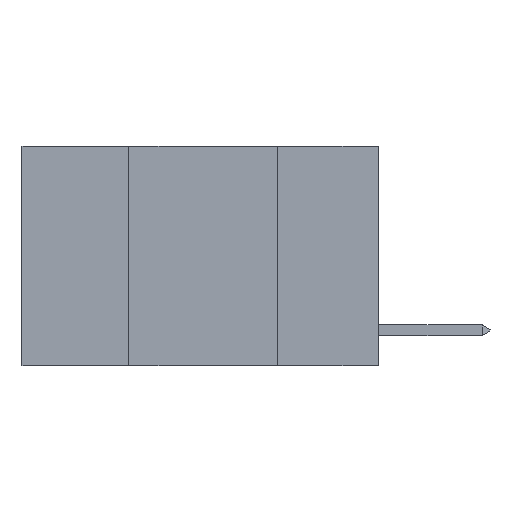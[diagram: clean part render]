
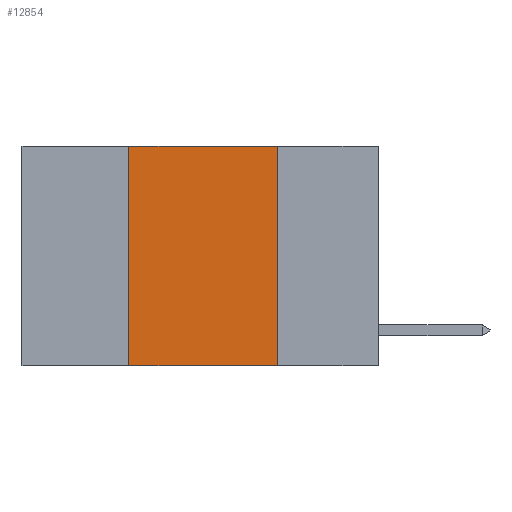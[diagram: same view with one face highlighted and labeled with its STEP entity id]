
A CAD part, left-side view. The second image highlights one B-rep face of the part: STEP entity #12854.
In plain terms, the highlighted planar face has unit normal (-1, 0, 0).
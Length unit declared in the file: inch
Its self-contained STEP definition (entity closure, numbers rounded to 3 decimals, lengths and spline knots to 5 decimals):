
#2386 = LINE ( 'NONE', #8048, #11723 ) ;
#2645 = VECTOR ( 'NONE', #6555, 39.37008 ) ;
#3430 = VERTEX_POINT ( 'NONE', #19271 ) ;
#3603 = VERTEX_POINT ( 'NONE', #8243 ) ;
#4232 = PLANE ( 'NONE',  #12462 ) ;
#4499 = ORIENTED_EDGE ( 'NONE', *, *, #13078, .F. ) ;
#5145 = VERTEX_POINT ( 'NONE', #18875 ) ;
#6231 = CARTESIAN_POINT ( 'NONE',  ( 0., 0.42, 0. ) ) ;
#6555 = DIRECTION ( 'NONE',  ( 0., -1., 0. ) ) ;
#6727 = VECTOR ( 'NONE', #12783, 39.37008 ) ;
#7423 = VECTOR ( 'NONE', #11514, 39.37008 ) ;
#7476 = EDGE_CURVE ( 'NONE', #3430, #5145, #15896, .T. ) ;
#7584 = CARTESIAN_POINT ( 'NONE',  ( 0., 0.6, 0. ) ) ;
#8048 = CARTESIAN_POINT ( 'NONE',  ( 0., 0.6, 0. ) ) ;
#8227 = CARTESIAN_POINT ( 'NONE',  ( 0., 0.6, -0.37 ) ) ;
#8243 = CARTESIAN_POINT ( 'NONE',  ( 0., 0.42, 0. ) ) ;
#8637 = EDGE_CURVE ( 'NONE', #3430, #3603, #18887, .T. ) ;
#9293 = DIRECTION ( 'NONE',  ( 0., 0., -1. ) ) ;
#9425 = ORIENTED_EDGE ( 'NONE', *, *, #16984, .F. ) ;
#11514 = DIRECTION ( 'NONE',  ( 0., 0., -1. ) ) ;
#11723 = VECTOR ( 'NONE', #17978, 39.37008 ) ;
#11873 = LINE ( 'NONE', #16446, #7423 ) ;
#12141 = FACE_OUTER_BOUND ( 'NONE', #12639, .T. ) ;
#12462 = AXIS2_PLACEMENT_3D ( 'NONE', #7584, #19152, #9293 ) ;
#12639 = EDGE_LOOP ( 'NONE', ( #4499, #9425, #13835, #18216 ) ) ;
#12783 = DIRECTION ( 'NONE',  ( 0., 0., 1. ) ) ;
#12854 = ADVANCED_FACE ( 'NONE', ( #12141 ), #4232, .F. ) ;
#13078 = EDGE_CURVE ( 'NONE', #17000, #5145, #11873, .T. ) ;
#13835 = ORIENTED_EDGE ( 'NONE', *, *, #8637, .F. ) ;
#14720 = CARTESIAN_POINT ( 'NONE',  ( 0., 0.17, 0. ) ) ;
#15896 = LINE ( 'NONE', #8227, #2645 ) ;
#16446 = CARTESIAN_POINT ( 'NONE',  ( 0., 0.17, 0. ) ) ;
#16984 = EDGE_CURVE ( 'NONE', #3603, #17000, #2386, .T. ) ;
#17000 = VERTEX_POINT ( 'NONE', #14720 ) ;
#17978 = DIRECTION ( 'NONE',  ( 0., -1., 0. ) ) ;
#18216 = ORIENTED_EDGE ( 'NONE', *, *, #7476, .T. ) ;
#18875 = CARTESIAN_POINT ( 'NONE',  ( 0., 0.17, -0.37 ) ) ;
#18887 = LINE ( 'NONE', #6231, #6727 ) ;
#19152 = DIRECTION ( 'NONE',  ( 1., 0., 0. ) ) ;
#19271 = CARTESIAN_POINT ( 'NONE',  ( 0., 0.42, -0.37 ) ) ;
